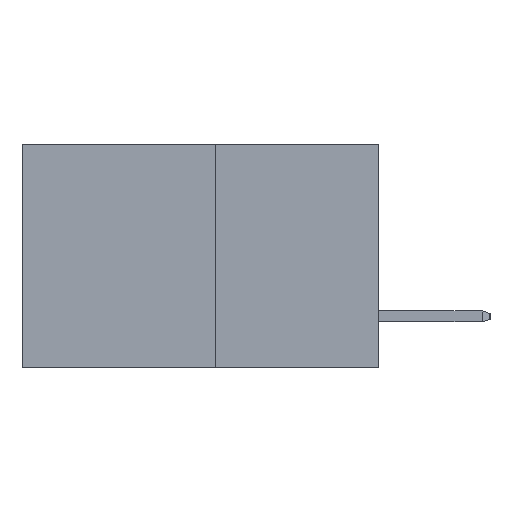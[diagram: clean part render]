
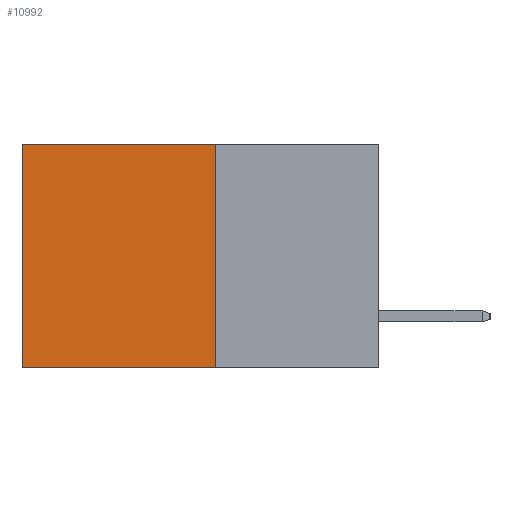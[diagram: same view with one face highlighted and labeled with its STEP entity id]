
A CAD part, left-side view. The second image highlights one B-rep face of the part: STEP entity #10992.
In plain terms, the highlighted planar face has unit normal (-1, 0, 0).
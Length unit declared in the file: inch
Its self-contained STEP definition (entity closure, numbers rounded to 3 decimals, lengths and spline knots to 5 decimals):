
#102 = EDGE_CURVE ( 'NONE', #6166, #2263, #12591, .T. ) ;
#2042 = VERTEX_POINT ( 'NONE', #20983 ) ;
#2263 = VERTEX_POINT ( 'NONE', #17870 ) ;
#2359 = VERTEX_POINT ( 'NONE', #11144 ) ;
#3984 = LINE ( 'NONE', #19502, #21573 ) ;
#5104 = LINE ( 'NONE', #11689, #9835 ) ;
#5445 = EDGE_CURVE ( 'NONE', #2042, #6166, #5104, .T. ) ;
#6119 = EDGE_CURVE ( 'NONE', #2042, #2359, #3984, .T. ) ;
#6166 = VERTEX_POINT ( 'NONE', #16676 ) ;
#6929 = PLANE ( 'NONE',  #8892 ) ;
#8667 = DIRECTION ( 'NONE',  ( 1., 0., 0. ) ) ;
#8892 = AXIS2_PLACEMENT_3D ( 'NONE', #17457, #8667, #20926 ) ;
#9835 = VECTOR ( 'NONE', #11609, 39.37008 ) ;
#10355 = EDGE_LOOP ( 'NONE', ( #17193, #17451, #18003, #18520 ) ) ;
#10670 = FACE_OUTER_BOUND ( 'NONE', #10355, .T. ) ;
#10992 = ADVANCED_FACE ( 'NONE', ( #10670 ), #6929, .F. ) ;
#11144 = CARTESIAN_POINT ( 'NONE',  ( 0.277, 0.59, 0. ) ) ;
#11609 = DIRECTION ( 'NONE',  ( 0., 0., -1. ) ) ;
#11689 = CARTESIAN_POINT ( 'NONE',  ( 0.277, 0.27, -0.37 ) ) ;
#12591 = LINE ( 'NONE', #13976, #21242 ) ;
#12634 = DIRECTION ( 'NONE',  ( 0., 0., -1. ) ) ;
#13976 = CARTESIAN_POINT ( 'NONE',  ( 0.277, 0.27, -0.37 ) ) ;
#16440 = DIRECTION ( 'NONE',  ( 0., 1., 0. ) ) ;
#16676 = CARTESIAN_POINT ( 'NONE',  ( 0.277, 0.27, -0.37 ) ) ;
#17193 = ORIENTED_EDGE ( 'NONE', *, *, #22843, .T. ) ;
#17451 = ORIENTED_EDGE ( 'NONE', *, *, #102, .F. ) ;
#17457 = CARTESIAN_POINT ( 'NONE',  ( 0.277, 0.27, -0.37 ) ) ;
#17870 = CARTESIAN_POINT ( 'NONE',  ( 0.277, 0.59, -0.37 ) ) ;
#17966 = VECTOR ( 'NONE', #12634, 39.37008 ) ;
#18003 = ORIENTED_EDGE ( 'NONE', *, *, #5445, .F. ) ;
#18520 = ORIENTED_EDGE ( 'NONE', *, *, #6119, .T. ) ;
#19232 = DIRECTION ( 'NONE',  ( 0., 1., 0. ) ) ;
#19502 = CARTESIAN_POINT ( 'NONE',  ( 0.277, 0.27, 0. ) ) ;
#20926 = DIRECTION ( 'NONE',  ( 0., 0., -1. ) ) ;
#20983 = CARTESIAN_POINT ( 'NONE',  ( 0.277, 0.27, 0. ) ) ;
#21242 = VECTOR ( 'NONE', #16440, 39.37008 ) ;
#21249 = CARTESIAN_POINT ( 'NONE',  ( 0.277, 0.59, -0.37 ) ) ;
#21442 = LINE ( 'NONE', #21249, #17966 ) ;
#21573 = VECTOR ( 'NONE', #19232, 39.37008 ) ;
#22843 = EDGE_CURVE ( 'NONE', #2359, #2263, #21442, .T. ) ;
